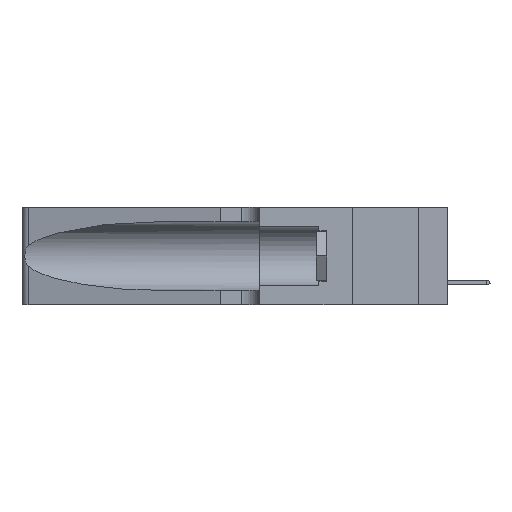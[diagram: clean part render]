
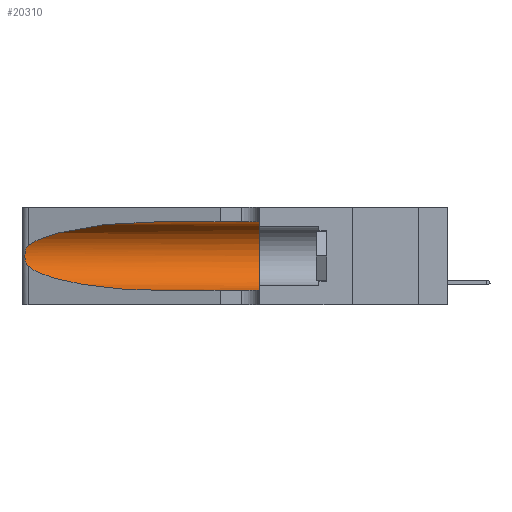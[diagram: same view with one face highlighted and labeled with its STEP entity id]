
A CAD part, left-side view. The second image highlights one B-rep face of the part: STEP entity #20310.
In plain terms, the highlighted cylindrical face has radius 3.308 mm (diameter 6.617 mm), a partial arc.
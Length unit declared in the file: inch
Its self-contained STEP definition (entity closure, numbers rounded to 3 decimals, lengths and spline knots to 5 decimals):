
#113 = FACE_OUTER_BOUND ( 'NONE', #43910, .T. ) ;
#386 = DIRECTION ( 'NONE',  ( 0., 1., 0. ) ) ;
#454 = ORIENTED_EDGE ( 'NONE', *, *, #4344, .F. ) ;
#643 = VERTEX_POINT ( 'NONE', #4704 ) ;
#961 = ORIENTED_EDGE ( 'NONE', *, *, #43820, .T. ) ;
#2690 = ORIENTED_EDGE ( 'NONE', *, *, #6901, .T. ) ;
#2920 = VERTEX_POINT ( 'NONE', #20655 ) ;
#3147 = CARTESIAN_POINT ( 'NONE',  ( 0.25854, 1.2359, 0.20912 ) ) ;
#3540 = CARTESIAN_POINT ( 'NONE',  ( 0.25639, 1.23186, 0.15144 ) ) ;
#3639 = CARTESIAN_POINT ( 'NONE',  ( 0.2373, 1.15595, 0.28018 ) ) ;
#4141 = CARTESIAN_POINT ( 'NONE',  ( 0.18966, 0.96281, 0.05475 ) ) ;
#4344 = EDGE_CURVE ( 'NONE', #643, #20283, #40559, .T. ) ;
#4493 = DIRECTION ( 'NONE',  ( 0., -1., 0. ) ) ;
#4567 = CARTESIAN_POINT ( 'NONE',  ( 0.1305, 0.35, 0.05475 ) ) ;
#4704 = CARTESIAN_POINT ( 'NONE',  ( 0.1305, 0.35, 0.31525 ) ) ;
#5070 = ORIENTED_EDGE ( 'NONE', *, *, #26401, .F. ) ;
#5554 = EDGE_CURVE ( 'NONE', #9523, #36593, #45034, .T. ) ;
#5998 = CARTESIAN_POINT ( 'NONE',  ( 0.1305, 1.61858, 0.31525 ) ) ;
#6901 = EDGE_CURVE ( 'NONE', #2920, #9523, #33435, .T. ) ;
#8074 = AXIS2_PLACEMENT_3D ( 'NONE', #39764, #36084, #18652 ) ;
#8858 = VECTOR ( 'NONE', #19064, 39.37008 ) ;
#9523 = VERTEX_POINT ( 'NONE', #36906 ) ;
#9941 = CARTESIAN_POINT ( 'NONE',  ( 0.26075, 1.23896, 0.178 ) ) ;
#10088 = CARTESIAN_POINT ( 'NONE',  ( 0.26017, 1.23833, 0.17102 ) ) ;
#10710 = CARTESIAN_POINT ( 'NONE',  ( 0.2373, 1.15595, 0.08982 ) ) ;
#10856 = CARTESIAN_POINT ( 'NONE',  ( 0.1305, 0.72297, 0.05475 ) ) ;
#10958 = CARTESIAN_POINT ( 'NONE',  ( 0.25555, 1.22993, 0.14849 ) ) ;
#12289 = CARTESIAN_POINT ( 'NONE',  ( 0.1305, 0.72297, 0.05475 ) ) ;
#12692 = AXIS2_PLACEMENT_3D ( 'NONE', #39443, #386, #25122 ) ;
#13496 = LINE ( 'NONE', #36794, #38831 ) ;
#14789 = CARTESIAN_POINT ( 'NONE',  ( 0.26075, 1.23896, 0.19203 ) ) ;
#18599 = CARTESIAN_POINT ( 'NONE',  ( 0.25487, 1.22718, 0.14631 ) ) ;
#18652 = DIRECTION ( 'NONE',  ( 0., 0., -1. ) ) ;
#19064 = DIRECTION ( 'NONE',  ( 0., -1., 0. ) ) ;
#20283 = VERTEX_POINT ( 'NONE', #4567 ) ;
#20310 = ADVANCED_FACE ( 'NONE', ( #113 ), #40399, .F. ) ;
#20655 = CARTESIAN_POINT ( 'NONE',  ( 0.1305, 0.72297, 0.31525 ) ) ;
#20881 = CARTESIAN_POINT ( 'NONE',  ( 0.25789, 1.23486, 0.15765 ) ) ;
#20917 = CARTESIAN_POINT ( 'NONE',  ( 0.25787, 1.23484, 0.2124 ) ) ;
#21311 = CARTESIAN_POINT ( 'NONE',  ( 0.25487, 1.22718, 0.14631 ) ) ;
#24295 = CARTESIAN_POINT ( 'NONE',  ( 0.25856, 1.23593, 0.16098 ) ) ;
#24972 = CARTESIAN_POINT ( 'NONE',  ( 0.18966, 0.96281, 0.31525 ) ) ;
#25122 = DIRECTION ( 'NONE',  ( 0., 0., 1. ) ) ;
#26401 = EDGE_CURVE ( 'NONE', #2920, #643, #26544, .T. ) ;
#26544 = LINE ( 'NONE', #5998, #8858 ) ;
#27734 = CARTESIAN_POINT ( 'NONE',  ( 0.25555, 1.22994, 0.2215 ) ) ;
#31559 = ORIENTED_EDGE ( 'NONE', *, *, #40564, .T. ) ;
#32384 = CARTESIAN_POINT ( 'NONE',  ( 0.25487, 1.22718, 0.22369 ) ) ;
#33435 =( BOUNDED_CURVE ( )  B_SPLINE_CURVE ( 3, ( #35751, #24972, #3639, #32384 ),
 .UNSPECIFIED., .F., .F. ) 
 B_SPLINE_CURVE_WITH_KNOTS ( ( 4, 4 ),
 ( 1.5708, 2.84003 ),
 .UNSPECIFIED. ) 
 CURVE ( )  GEOMETRIC_REPRESENTATION_ITEM ( )  RATIONAL_B_SPLINE_CURVE ( ( 1., 0.87, 0.87, 1. ) ) 
 REPRESENTATION_ITEM ( '' )  );
#34829 = CARTESIAN_POINT ( 'NONE',  ( 0.25639, 1.23184, 0.21858 ) ) ;
#35751 = CARTESIAN_POINT ( 'NONE',  ( 0.1305, 0.72297, 0.31525 ) ) ;
#36084 = DIRECTION ( 'NONE',  ( 0., -1., 0. ) ) ;
#36593 = VERTEX_POINT ( 'NONE', #18599 ) ;
#36794 = CARTESIAN_POINT ( 'NONE',  ( 0.1305, 1.61858, 0.05475 ) ) ;
#36906 = CARTESIAN_POINT ( 'NONE',  ( 0.25487, 1.22718, 0.22369 ) ) ;
#37374 =( BOUNDED_CURVE ( )  B_SPLINE_CURVE ( 3, ( #38766, #10710, #4141, #10856 ),
 .UNSPECIFIED., .F., .T. ) 
 B_SPLINE_CURVE_WITH_KNOTS ( ( 4, 4 ),
 ( 3.44316, 4.71239 ),
 .UNSPECIFIED. ) 
 CURVE ( )  GEOMETRIC_REPRESENTATION_ITEM ( )  RATIONAL_B_SPLINE_CURVE ( ( 1., 0.87, 0.87, 1. ) ) 
 REPRESENTATION_ITEM ( '' )  );
#38766 = CARTESIAN_POINT ( 'NONE',  ( 0.25487, 1.22718, 0.14631 ) ) ;
#38831 = VECTOR ( 'NONE', #4493, 39.37008 ) ;
#39443 = CARTESIAN_POINT ( 'NONE',  ( 0.1305, 0.35, 0.185 ) ) ;
#39764 = CARTESIAN_POINT ( 'NONE',  ( 0.1305, 1.61858, 0.185 ) ) ;
#40399 = CYLINDRICAL_SURFACE ( 'NONE', #8074, 0.13025 ) ;
#40559 = CIRCLE ( 'NONE', #12692, 0.13025 ) ;
#40564 = EDGE_CURVE ( 'NONE', #36593, #42462, #37374, .T. ) ;
#41829 = ORIENTED_EDGE ( 'NONE', *, *, #5554, .T. ) ;
#42462 = VERTEX_POINT ( 'NONE', #12289 ) ;
#42473 = CARTESIAN_POINT ( 'NONE',  ( 0.25487, 1.22718, 0.22369 ) ) ;
#43820 = EDGE_CURVE ( 'NONE', #42462, #20283, #13496, .T. ) ;
#43910 = EDGE_LOOP ( 'NONE', ( #2690, #41829, #31559, #961, #454, #5070 ) ) ;
#45034 = B_SPLINE_CURVE_WITH_KNOTS ( 'NONE', 3,
 ( #42473, #27734, #34829, #20917, #3147, #45592, #14789, #9941, #10088, #24295, #20881, #3540, #10958, #21311 ),
 .UNSPECIFIED., .F., .F.,
 ( 4, 2, 2, 2, 2, 2, 4 ),
 ( 0., 0.00027, 0.00053, 0.00107, 0.0016, 0.00187, 0.00214 ),
 .UNSPECIFIED. ) ;
#45592 = CARTESIAN_POINT ( 'NONE',  ( 0.26018, 1.23835, 0.19895 ) ) ;
